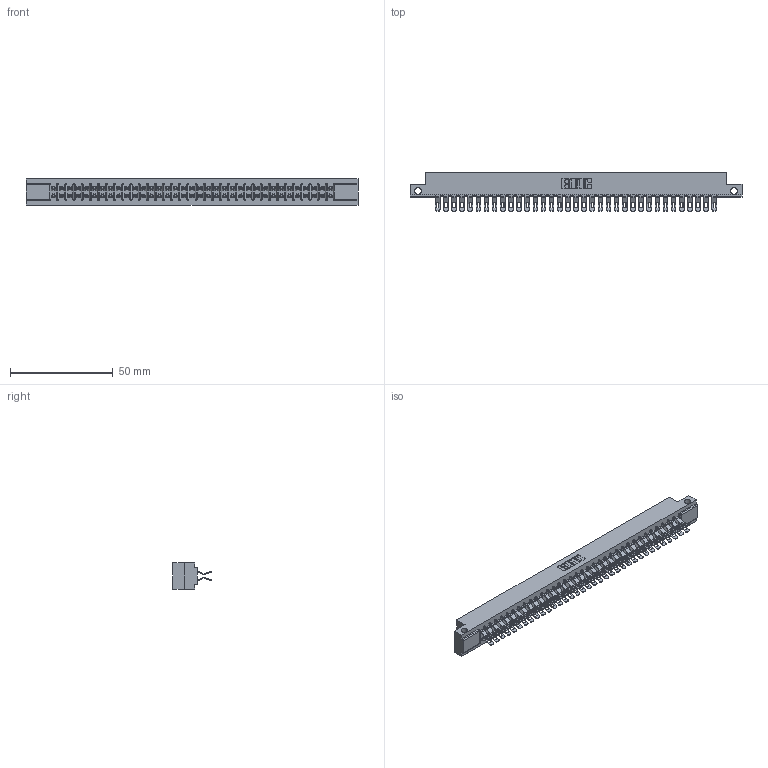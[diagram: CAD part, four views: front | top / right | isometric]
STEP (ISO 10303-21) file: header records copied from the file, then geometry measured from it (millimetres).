
FILE_DESCRIPTION (( 'STEP AP203' ), '1' );
FILE_NAME ('357-070-555-212.STEP', '2019-09-19T10:37:40', ( '' ), ( '' ), 'SwSTEP 2.0', 'SolidWorks 2016', '' );
FILE_SCHEMA (( 'CONFIG_CONTROL_DESIGN' ));
Length unit declared in the file: inch
Products named in the file (3): 307 Part_.128 Dia Side Mounting Holes; 357-070-555-212; 307-290-001_555
Assembly tree (71 placements, depth 2):
  357-070-555-212
    307 Part_.128 Dia Side Mounting Holes
    307-290-001_555  x70
Bounding box: 161.7 x 18.75 x 12.7 mm (x, y, z)
Volume: 17211.3 mm3; surface area: 22060.8 mm2
Topology: 71 solids, 71 shells, 4424 faces, 12993 edges, 8470 vertices
Faces by surface type: plane 2450, cylinder 1902, sphere 72
Entity records: 32527 total; most frequent: CARTESIAN_POINT 5327, ORIENTED_EDGE 5280, DIRECTION 5228, EDGE_CURVE 2640, VECTOR 2010, LINE 2010, VERTEX_POINT 1708, AXIS2_PLACEMENT_3D 1609
